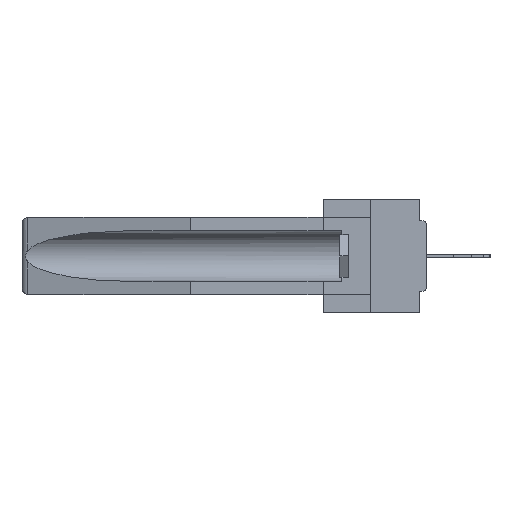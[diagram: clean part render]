
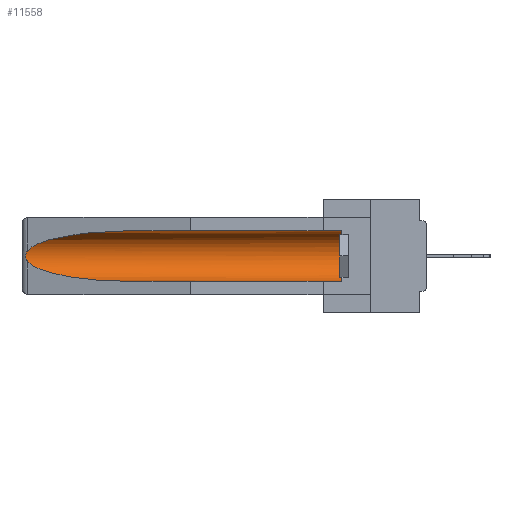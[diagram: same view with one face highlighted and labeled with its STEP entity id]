
A CAD part, left-side view. The second image highlights one B-rep face of the part: STEP entity #11558.
In plain terms, the highlighted cylindrical face has radius 2.857 mm (diameter 5.715 mm), a partial arc.
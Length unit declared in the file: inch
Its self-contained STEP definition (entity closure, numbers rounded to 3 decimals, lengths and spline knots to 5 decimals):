
#13 = CARTESIAN_POINT ( 'NONE',  ( 0.155, 1.07973, -0.059 ) ) ;
#954 = B_SPLINE_CURVE_WITH_KNOTS ( 'NONE', 3,
 ( #16624, #29598, #19201, #3555, #21835, #6210, #24439, #8862, #27056, #11483 ),
 .UNSPECIFIED., .F., .F.,
 ( 4, 2, 2, 2, 4 ),
 ( 0., 0.00029, 0.00058, 0.00087, 0.00117 ),
 .UNSPECIFIED. ) ;
#1830 = EDGE_CURVE ( 'NONE', #21410, #18302, #24035, .T. ) ;
#2813 = ORIENTED_EDGE ( 'NONE', *, *, #1830, .T. ) ;
#3393 = CARTESIAN_POINT ( 'NONE',  ( 0.155, 1.07973, -0.284 ) ) ;
#3457 = CARTESIAN_POINT ( 'NONE',  ( 0.25451, 1.48313, -0.24835 ) ) ;
#3555 = CARTESIAN_POINT ( 'NONE',  ( 0.2673, 1.5327, -0.16383 ) ) ;
#3765 = ORIENTED_EDGE ( 'NONE', *, *, #25211, .T. ) ;
#3958 = ORIENTED_EDGE ( 'NONE', *, *, #21729, .T. ) ;
#6210 = CARTESIAN_POINT ( 'NONE',  ( 0.2675, 1.53308, -0.17534 ) ) ;
#7373 = EDGE_CURVE ( 'NONE', #10623, #22988, #9553, .T. ) ;
#7852 = LINE ( 'NONE', #16295, #13965 ) ;
#8074 = DIRECTION ( 'NONE',  ( 0., 0., 1. ) ) ;
#8862 = CARTESIAN_POINT ( 'NONE',  ( 0.26655, 1.53094, -0.18657 ) ) ;
#9553 =( BOUNDED_CURVE ( )  B_SPLINE_CURVE ( 3, ( #26954, #3457, #11380, #14007 ),
 .UNSPECIFIED., .F., .F. ) 
 B_SPLINE_CURVE_WITH_KNOTS ( ( 4, 4 ),
 ( 0.1948, 1.5708 ),
 .UNSPECIFIED. ) 
 CURVE ( )  GEOMETRIC_REPRESENTATION_ITEM ( )  RATIONAL_B_SPLINE_CURVE ( ( 1., 0.848, 0.848, 1. ) ) 
 REPRESENTATION_ITEM ( '' )  );
#9906 = CARTESIAN_POINT ( 'NONE',  ( 0.25451, 1.48313, -0.09465 ) ) ;
#10567 = VERTEX_POINT ( 'NONE', #31300 ) ;
#10576 = CARTESIAN_POINT ( 'NONE',  ( 0.26537, 1.52718, -0.19328 ) ) ;
#10623 = VERTEX_POINT ( 'NONE', #10576 ) ;
#10641 = CARTESIAN_POINT ( 'NONE',  ( 0.155, 0.126, -0.059 ) ) ;
#10662 = DIRECTION ( 'NONE',  ( 0., 1., 0. ) ) ;
#11024 = DIRECTION ( 'NONE',  ( 0., 1., 0. ) ) ;
#11380 = CARTESIAN_POINT ( 'NONE',  ( 0.21114, 1.30732, -0.284 ) ) ;
#11483 = CARTESIAN_POINT ( 'NONE',  ( 0.26537, 1.52718, -0.19328 ) ) ;
#11558 = ADVANCED_FACE ( 'NONE', ( #19618 ), #31831, .F. ) ;
#13334 = CIRCLE ( 'NONE', #14109, 0.1125 ) ;
#13965 = VECTOR ( 'NONE', #11024, 39.37008 ) ;
#14007 = CARTESIAN_POINT ( 'NONE',  ( 0.155, 1.07973, -0.284 ) ) ;
#14109 = AXIS2_PLACEMENT_3D ( 'NONE', #30226, #14642, #32823 ) ;
#14642 = DIRECTION ( 'NONE',  ( 0., -1., 0. ) ) ;
#15281 = VERTEX_POINT ( 'NONE', #27655 ) ;
#15392 =( BOUNDED_CURVE ( )  B_SPLINE_CURVE ( 3, ( #20278, #33231, #9906, #28145 ),
 .UNSPECIFIED., .F., .F. ) 
 B_SPLINE_CURVE_WITH_KNOTS ( ( 4, 4 ),
 ( 4.71239, 6.08839 ),
 .UNSPECIFIED. ) 
 CURVE ( )  GEOMETRIC_REPRESENTATION_ITEM ( )  RATIONAL_B_SPLINE_CURVE ( ( 1., 0.848, 0.848, 1. ) ) 
 REPRESENTATION_ITEM ( '' )  );
#16295 = CARTESIAN_POINT ( 'NONE',  ( 0.155, -0.30754, -0.284 ) ) ;
#16624 = CARTESIAN_POINT ( 'NONE',  ( 0.26537, 1.52718, -0.14972 ) ) ;
#18302 = VERTEX_POINT ( 'NONE', #13 ) ;
#19201 = CARTESIAN_POINT ( 'NONE',  ( 0.26654, 1.53092, -0.15636 ) ) ;
#19618 = FACE_OUTER_BOUND ( 'NONE', #27141, .T. ) ;
#19626 = ORIENTED_EDGE ( 'NONE', *, *, #31005, .T. ) ;
#20278 = CARTESIAN_POINT ( 'NONE',  ( 0.155, 1.07973, -0.059 ) ) ;
#21410 = VERTEX_POINT ( 'NONE', #10641 ) ;
#21729 = EDGE_CURVE ( 'NONE', #15281, #21410, #13334, .T. ) ;
#21835 = CARTESIAN_POINT ( 'NONE',  ( 0.2675, 1.53308, -0.16763 ) ) ;
#22988 = VERTEX_POINT ( 'NONE', #3393 ) ;
#23215 = VECTOR ( 'NONE', #29214, 39.37008 ) ;
#24035 = LINE ( 'NONE', #27980, #23215 ) ;
#24439 = CARTESIAN_POINT ( 'NONE',  ( 0.2673, 1.53269, -0.17917 ) ) ;
#25211 = EDGE_CURVE ( 'NONE', #10567, #10623, #954, .T. ) ;
#26253 = CARTESIAN_POINT ( 'NONE',  ( 0.155, -0.30754, -0.1715 ) ) ;
#26951 = EDGE_CURVE ( 'NONE', #15281, #22988, #7852, .T. ) ;
#26954 = CARTESIAN_POINT ( 'NONE',  ( 0.26537, 1.52718, -0.19328 ) ) ;
#27056 = CARTESIAN_POINT ( 'NONE',  ( 0.26597, 1.5296, -0.19026 ) ) ;
#27141 = EDGE_LOOP ( 'NONE', ( #19626, #3765, #29989, #29228, #3958, #2813 ) ) ;
#27655 = CARTESIAN_POINT ( 'NONE',  ( 0.155, 0.126, -0.284 ) ) ;
#27980 = CARTESIAN_POINT ( 'NONE',  ( 0.155, -0.30754, -0.059 ) ) ;
#28145 = CARTESIAN_POINT ( 'NONE',  ( 0.26537, 1.52718, -0.14972 ) ) ;
#29214 = DIRECTION ( 'NONE',  ( 0., 1., 0. ) ) ;
#29228 = ORIENTED_EDGE ( 'NONE', *, *, #26951, .F. ) ;
#29598 = CARTESIAN_POINT ( 'NONE',  ( 0.26597, 1.52961, -0.15275 ) ) ;
#29989 = ORIENTED_EDGE ( 'NONE', *, *, #7373, .T. ) ;
#30024 = AXIS2_PLACEMENT_3D ( 'NONE', #26253, #10662, #8074 ) ;
#30226 = CARTESIAN_POINT ( 'NONE',  ( 0.155, 0.126, -0.1715 ) ) ;
#31005 = EDGE_CURVE ( 'NONE', #18302, #10567, #15392, .T. ) ;
#31300 = CARTESIAN_POINT ( 'NONE',  ( 0.26537, 1.52718, -0.14972 ) ) ;
#31831 = CYLINDRICAL_SURFACE ( 'NONE', #30024, 0.1125 ) ;
#32823 = DIRECTION ( 'NONE',  ( 0., 0., 1. ) ) ;
#33231 = CARTESIAN_POINT ( 'NONE',  ( 0.21114, 1.30732, -0.059 ) ) ;
